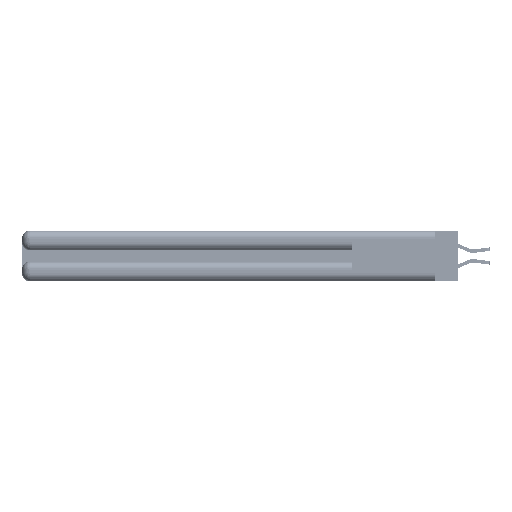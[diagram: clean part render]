
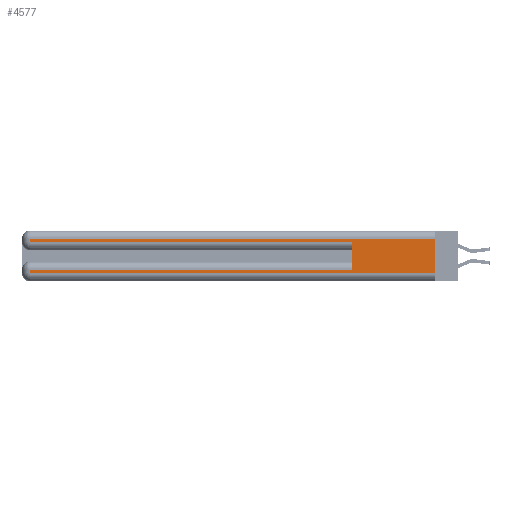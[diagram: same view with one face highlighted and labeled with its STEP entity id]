
A CAD part, left-side view. The second image highlights one B-rep face of the part: STEP entity #4577.
In plain terms, the highlighted planar face has unit normal (-1, 0, 0).
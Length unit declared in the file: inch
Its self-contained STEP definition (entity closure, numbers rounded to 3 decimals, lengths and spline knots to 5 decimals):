
#453 = LINE ( 'NONE', #8675, #47872 ) ;
#1217 = CARTESIAN_POINT ( 'NONE',  ( 0., 0.6, 0.145 ) ) ;
#1325 = CARTESIAN_POINT ( 'NONE',  ( 0., 0., 0.285 ) ) ;
#1661 = DIRECTION ( 'NONE',  ( 1., 0., 0. ) ) ;
#1949 = ORIENTED_EDGE ( 'NONE', *, *, #45325, .F. ) ;
#3223 = CARTESIAN_POINT ( 'NONE',  ( 0., 0., 0.37 ) ) ;
#4577 = ADVANCED_FACE ( 'NONE', ( #33085 ), #17826, .F. ) ;
#6283 = LINE ( 'NONE', #32035, #30316 ) ;
#8675 = CARTESIAN_POINT ( 'NONE',  ( 0., 2.94, 0.37 ) ) ;
#9040 = ORIENTED_EDGE ( 'NONE', *, *, #14998, .T. ) ;
#10249 = DIRECTION ( 'NONE',  ( 0., -1., 0. ) ) ;
#10632 = VERTEX_POINT ( 'NONE', #28193 ) ;
#10713 = EDGE_CURVE ( 'NONE', #30801, #44909, #47098, .T. ) ;
#10768 = CARTESIAN_POINT ( 'NONE',  ( 0., 2.94, 0.37 ) ) ;
#12498 = VECTOR ( 'NONE', #36475, 39.37008 ) ;
#12985 = VECTOR ( 'NONE', #42755, 39.37008 ) ;
#13062 = VECTOR ( 'NONE', #20555, 39.37008 ) ;
#14935 = DIRECTION ( 'NONE',  ( 0., 0., -1. ) ) ;
#14998 = EDGE_CURVE ( 'NONE', #22881, #39122, #453, .T. ) ;
#15552 = CARTESIAN_POINT ( 'NONE',  ( 0., 2.94, 0.085 ) ) ;
#16968 = ORIENTED_EDGE ( 'NONE', *, *, #41815, .T. ) ;
#17655 = DIRECTION ( 'NONE',  ( 0., 0., -1. ) ) ;
#17826 = PLANE ( 'NONE',  #34173 ) ;
#18436 = ORIENTED_EDGE ( 'NONE', *, *, #36666, .T. ) ;
#18545 = LINE ( 'NONE', #10768, #12985 ) ;
#18556 = EDGE_CURVE ( 'NONE', #36623, #44909, #33353, .T. ) ;
#19818 = DIRECTION ( 'NONE',  ( 0., 1., 0. ) ) ;
#20555 = DIRECTION ( 'NONE',  ( 0., 1., 0. ) ) ;
#20701 = DIRECTION ( 'NONE',  ( 0., 0., -1. ) ) ;
#22881 = VERTEX_POINT ( 'NONE', #15552 ) ;
#28193 = CARTESIAN_POINT ( 'NONE',  ( 0., 0., 0.06 ) ) ;
#28692 = VECTOR ( 'NONE', #14935, 39.37008 ) ;
#28803 = CARTESIAN_POINT ( 'NONE',  ( 0., 0., 0.31 ) ) ;
#30316 = VECTOR ( 'NONE', #19818, 39.37008 ) ;
#30528 = ORIENTED_EDGE ( 'NONE', *, *, #18556, .F. ) ;
#30801 = VERTEX_POINT ( 'NONE', #31902 ) ;
#31532 = LINE ( 'NONE', #28803, #13062 ) ;
#31902 = CARTESIAN_POINT ( 'NONE',  ( 0., 2.94, 0.285 ) ) ;
#32035 = CARTESIAN_POINT ( 'NONE',  ( 0., 0., 0.085 ) ) ;
#32502 = EDGE_CURVE ( 'NONE', #35007, #30801, #18545, .T. ) ;
#33085 = FACE_OUTER_BOUND ( 'NONE', #33921, .T. ) ;
#33353 = LINE ( 'NONE', #1217, #12498 ) ;
#33921 = EDGE_LOOP ( 'NONE', ( #1949, #16968, #38948, #48073, #30528, #18436, #9040, #41033 ) ) ;
#34173 = AXIS2_PLACEMENT_3D ( 'NONE', #41215, #1661, #17655 ) ;
#35007 = VERTEX_POINT ( 'NONE', #41832 ) ;
#36475 = DIRECTION ( 'NONE',  ( 0., 0., 1. ) ) ;
#36621 = VECTOR ( 'NONE', #44533, 39.37008 ) ;
#36623 = VERTEX_POINT ( 'NONE', #43054 ) ;
#36666 = EDGE_CURVE ( 'NONE', #36623, #22881, #6283, .T. ) ;
#37620 = EDGE_CURVE ( 'NONE', #39122, #10632, #39413, .T. ) ;
#38948 = ORIENTED_EDGE ( 'NONE', *, *, #32502, .T. ) ;
#39122 = VERTEX_POINT ( 'NONE', #44040 ) ;
#39138 = LINE ( 'NONE', #3223, #28692 ) ;
#39413 = LINE ( 'NONE', #41377, #48086 ) ;
#41033 = ORIENTED_EDGE ( 'NONE', *, *, #37620, .T. ) ;
#41215 = CARTESIAN_POINT ( 'NONE',  ( 0., 0., 0.37 ) ) ;
#41377 = CARTESIAN_POINT ( 'NONE',  ( 0., 0., 0.06 ) ) ;
#41815 = EDGE_CURVE ( 'NONE', #45082, #35007, #31532, .T. ) ;
#41832 = CARTESIAN_POINT ( 'NONE',  ( 0., 2.94, 0.31 ) ) ;
#42755 = DIRECTION ( 'NONE',  ( 0., 0., -1. ) ) ;
#43054 = CARTESIAN_POINT ( 'NONE',  ( 0., 0.6, 0.085 ) ) ;
#44040 = CARTESIAN_POINT ( 'NONE',  ( 0., 2.94, 0.06 ) ) ;
#44290 = CARTESIAN_POINT ( 'NONE',  ( 0., 0.6, 0.285 ) ) ;
#44533 = DIRECTION ( 'NONE',  ( 0., -1., 0. ) ) ;
#44909 = VERTEX_POINT ( 'NONE', #44290 ) ;
#45082 = VERTEX_POINT ( 'NONE', #49657 ) ;
#45325 = EDGE_CURVE ( 'NONE', #45082, #10632, #39138, .T. ) ;
#47098 = LINE ( 'NONE', #1325, #36621 ) ;
#47872 = VECTOR ( 'NONE', #20701, 39.37008 ) ;
#48073 = ORIENTED_EDGE ( 'NONE', *, *, #10713, .T. ) ;
#48086 = VECTOR ( 'NONE', #10249, 39.37008 ) ;
#49657 = CARTESIAN_POINT ( 'NONE',  ( 0., 0., 0.31 ) ) ;
